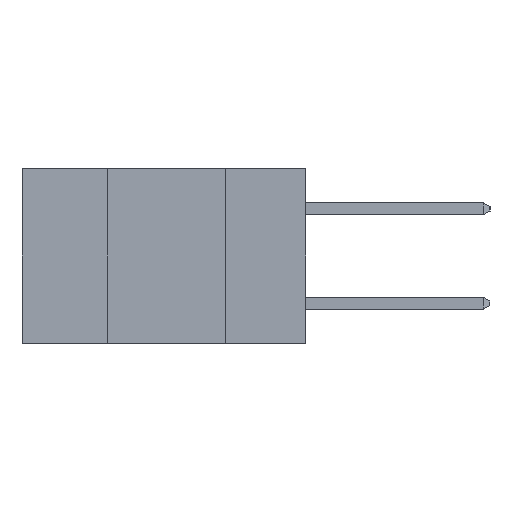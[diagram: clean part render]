
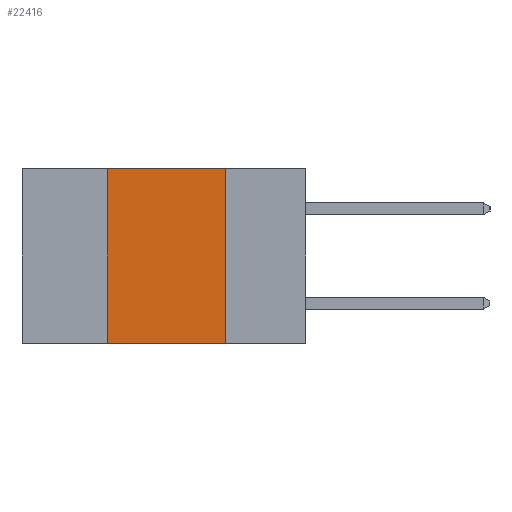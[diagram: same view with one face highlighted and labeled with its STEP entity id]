
A CAD part, left-side view. The second image highlights one B-rep face of the part: STEP entity #22416.
In plain terms, the highlighted planar face has unit normal (-1, 0, 0).
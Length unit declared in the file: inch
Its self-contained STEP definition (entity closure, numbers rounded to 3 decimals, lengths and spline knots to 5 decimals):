
#145 = DIRECTION ( 'NONE',  ( 0., 0., -1. ) ) ;
#160 = DIRECTION ( 'NONE',  ( 0., 0., 1. ) ) ;
#712 = VECTOR ( 'NONE', #160, 39.37008 ) ;
#1197 = VERTEX_POINT ( 'NONE', #22893 ) ;
#4374 = EDGE_CURVE ( 'NONE', #8582, #14152, #13973, .T. ) ;
#5597 = DIRECTION ( 'NONE',  ( 0., -1., 0. ) ) ;
#5839 = DIRECTION ( 'NONE',  ( 0., -1., 0. ) ) ;
#5858 = CARTESIAN_POINT ( 'NONE',  ( 0., 0.6, -0.37 ) ) ;
#7029 = VECTOR ( 'NONE', #5597, 39.37008 ) ;
#7439 = PLANE ( 'NONE',  #15455 ) ;
#8582 = VERTEX_POINT ( 'NONE', #9017 ) ;
#9017 = CARTESIAN_POINT ( 'NONE',  ( 0., 0.17, 0. ) ) ;
#9969 = EDGE_CURVE ( 'NONE', #15731, #14152, #12742, .T. ) ;
#10360 = LINE ( 'NONE', #21537, #712 ) ;
#11027 = DIRECTION ( 'NONE',  ( 1., 0., 0. ) ) ;
#12072 = CARTESIAN_POINT ( 'NONE',  ( 0., 0.17, -0.37 ) ) ;
#12197 = VECTOR ( 'NONE', #5839, 39.37008 ) ;
#12742 = LINE ( 'NONE', #5858, #12197 ) ;
#13673 = FACE_OUTER_BOUND ( 'NONE', #22118, .T. ) ;
#13973 = LINE ( 'NONE', #21932, #22713 ) ;
#14152 = VERTEX_POINT ( 'NONE', #12072 ) ;
#15455 = AXIS2_PLACEMENT_3D ( 'NONE', #21524, #11027, #145 ) ;
#15731 = VERTEX_POINT ( 'NONE', #21231 ) ;
#16782 = ORIENTED_EDGE ( 'NONE', *, *, #20985, .F. ) ;
#18379 = ORIENTED_EDGE ( 'NONE', *, *, #9969, .T. ) ;
#18614 = EDGE_CURVE ( 'NONE', #15731, #1197, #10360, .T. ) ;
#19658 = CARTESIAN_POINT ( 'NONE',  ( 0., 0.6, 0. ) ) ;
#20985 = EDGE_CURVE ( 'NONE', #1197, #8582, #21096, .T. ) ;
#21096 = LINE ( 'NONE', #19658, #7029 ) ;
#21231 = CARTESIAN_POINT ( 'NONE',  ( 0., 0.42, -0.37 ) ) ;
#21430 = ORIENTED_EDGE ( 'NONE', *, *, #4374, .F. ) ;
#21524 = CARTESIAN_POINT ( 'NONE',  ( 0., 0.6, 0. ) ) ;
#21537 = CARTESIAN_POINT ( 'NONE',  ( 0., 0.42, -0.37 ) ) ;
#21853 = DIRECTION ( 'NONE',  ( 0., 0., -1. ) ) ;
#21932 = CARTESIAN_POINT ( 'NONE',  ( 0., 0.17, -0.37 ) ) ;
#22118 = EDGE_LOOP ( 'NONE', ( #21430, #16782, #22260, #18379 ) ) ;
#22260 = ORIENTED_EDGE ( 'NONE', *, *, #18614, .F. ) ;
#22416 = ADVANCED_FACE ( 'NONE', ( #13673 ), #7439, .F. ) ;
#22713 = VECTOR ( 'NONE', #21853, 39.37008 ) ;
#22893 = CARTESIAN_POINT ( 'NONE',  ( 0., 0.42, 0. ) ) ;
